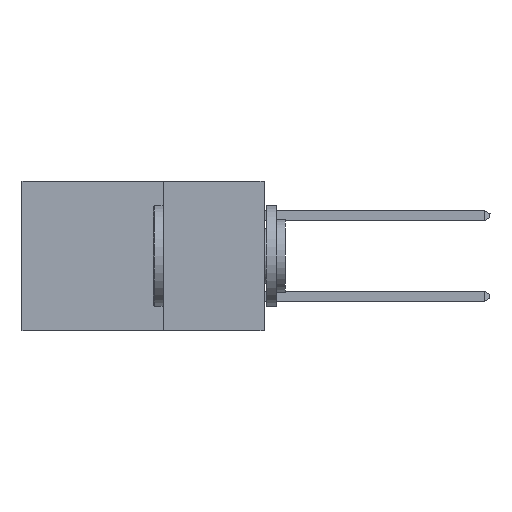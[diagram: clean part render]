
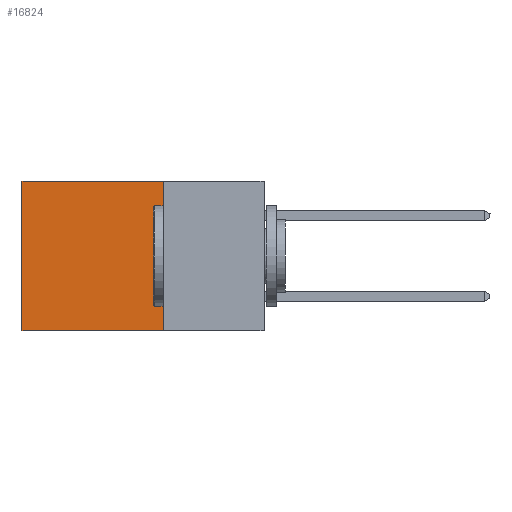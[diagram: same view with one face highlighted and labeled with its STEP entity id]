
A CAD part, left-side view. The second image highlights one B-rep face of the part: STEP entity #16824.
In plain terms, the highlighted planar face has unit normal (-1, 0, 0).
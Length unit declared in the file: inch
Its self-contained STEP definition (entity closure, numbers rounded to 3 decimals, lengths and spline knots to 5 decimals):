
#89 = CARTESIAN_POINT ( 'NONE',  ( 0.298, 0.6, 0. ) ) ;
#1397 = CARTESIAN_POINT ( 'NONE',  ( 0.298, 0.25, 0. ) ) ;
#1425 = EDGE_CURVE ( 'NONE', #23741, #21566, #11370, .T. ) ;
#1547 = EDGE_CURVE ( 'NONE', #1882, #21566, #15999, .T. ) ;
#1882 = VERTEX_POINT ( 'NONE', #10741 ) ;
#2091 = VECTOR ( 'NONE', #14514, 39.37008 ) ;
#3164 = DIRECTION ( 'NONE',  ( 1., 0., 0. ) ) ;
#5234 = VECTOR ( 'NONE', #7584, 39.37008 ) ;
#6116 = DIRECTION ( 'NONE',  ( 0., 0., -1. ) ) ;
#7239 = DIRECTION ( 'NONE',  ( 0., 0., -1. ) ) ;
#7387 = CARTESIAN_POINT ( 'NONE',  ( 0.298, 0.25, 0. ) ) ;
#7584 = DIRECTION ( 'NONE',  ( 0., 1., 0. ) ) ;
#8161 = VERTEX_POINT ( 'NONE', #7387 ) ;
#8567 = ORIENTED_EDGE ( 'NONE', *, *, #18730, .T. ) ;
#8817 = DIRECTION ( 'NONE',  ( 0., 0., -1. ) ) ;
#9268 = CARTESIAN_POINT ( 'NONE',  ( 0.298, 0.25, 0. ) ) ;
#10132 = AXIS2_PLACEMENT_3D ( 'NONE', #14084, #3164, #8817 ) ;
#10741 = CARTESIAN_POINT ( 'NONE',  ( 0.298, 0.6, 0. ) ) ;
#11370 = LINE ( 'NONE', #14793, #5234 ) ;
#11857 = CARTESIAN_POINT ( 'NONE',  ( 0.298, 0.25, -0.37 ) ) ;
#12544 = EDGE_LOOP ( 'NONE', ( #21633, #22817, #21771, #8567 ) ) ;
#13964 = VECTOR ( 'NONE', #6116, 39.37008 ) ;
#13979 = LINE ( 'NONE', #1397, #19825 ) ;
#14084 = CARTESIAN_POINT ( 'NONE',  ( 0.298, 0.25, 0. ) ) ;
#14102 = FACE_OUTER_BOUND ( 'NONE', #12544, .T. ) ;
#14514 = DIRECTION ( 'NONE',  ( 0., 1., 0. ) ) ;
#14793 = CARTESIAN_POINT ( 'NONE',  ( 0.298, 0.25, -0.37 ) ) ;
#15999 = LINE ( 'NONE', #89, #13964 ) ;
#16824 = ADVANCED_FACE ( 'NONE', ( #14102 ), #17844, .F. ) ;
#17844 = PLANE ( 'NONE',  #10132 ) ;
#18730 = EDGE_CURVE ( 'NONE', #8161, #1882, #23152, .T. ) ;
#19668 = CARTESIAN_POINT ( 'NONE',  ( 0.298, 0.6, -0.37 ) ) ;
#19825 = VECTOR ( 'NONE', #7239, 39.37008 ) ;
#21566 = VERTEX_POINT ( 'NONE', #19668 ) ;
#21633 = ORIENTED_EDGE ( 'NONE', *, *, #1547, .T. ) ;
#21771 = ORIENTED_EDGE ( 'NONE', *, *, #22830, .F. ) ;
#22817 = ORIENTED_EDGE ( 'NONE', *, *, #1425, .F. ) ;
#22830 = EDGE_CURVE ( 'NONE', #8161, #23741, #13979, .T. ) ;
#23152 = LINE ( 'NONE', #9268, #2091 ) ;
#23741 = VERTEX_POINT ( 'NONE', #11857 ) ;
